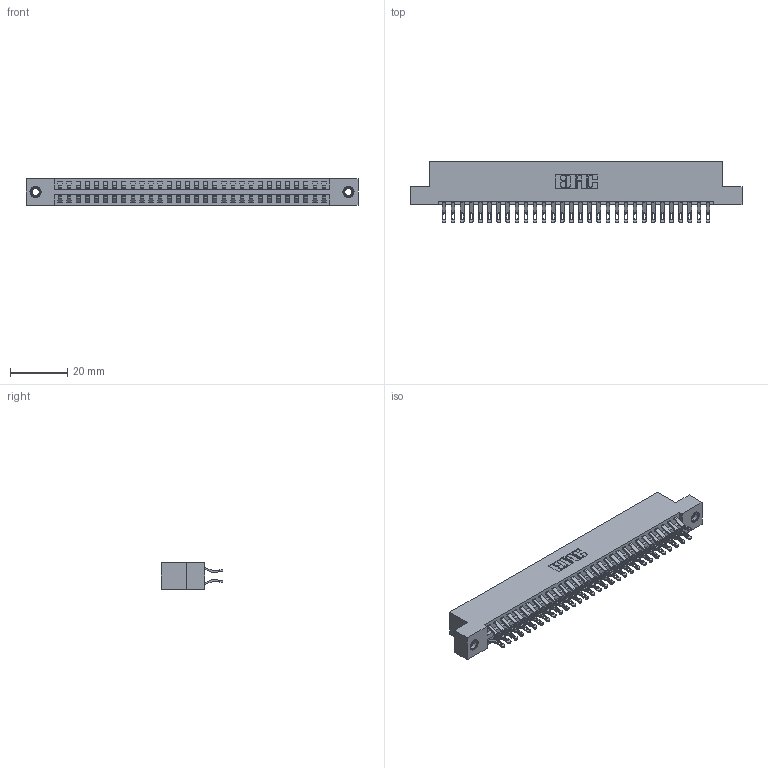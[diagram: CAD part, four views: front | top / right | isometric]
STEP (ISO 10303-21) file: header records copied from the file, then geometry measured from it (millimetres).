
FILE_DESCRIPTION (( 'STEP AP203' ), '1' );
FILE_NAME ('396-060-555-207.STEP', '2019-10-30T16:47:29', ( '' ), ( '' ), 'SwSTEP 2.0', 'SolidWorks 2016', '' );
FILE_SCHEMA (( 'CONFIG_CONTROL_DESIGN' ));
Length unit declared in the file: inch
Products named in the file (4): 396-060-555-207; 345-250-001_345-250-005-103; 345-292-001_555 Tail; 346 Part_Flush Mounting Lugs - 0.156 Dia-TI
Assembly tree (63 placements, depth 2):
  396-060-555-207
    346 Part_Flush Mounting Lugs - 0.156 Dia-TI
    345-292-001_555 Tail  x60
    345-250-001_345-250-005-103  x2
Bounding box: 115.82 x 21.46 x 9.4 mm (x, y, z)
Volume: 11361.6 mm3; surface area: 16082.8 mm2
Topology: 63 solids, 63 shells, 3662 faces, 11445 edges, 7622 vertices
Faces by surface type: plane 2088, cylinder 1558, cone 12, torus 4
Entity records: 22706 total; most frequent: CARTESIAN_POINT 3777, ORIENTED_EDGE 3674, DIRECTION 3375, EDGE_CURVE 1837, LINE 1545, VECTOR 1545, VERTEX_POINT 1220, AXIS2_PLACEMENT_3D 915
